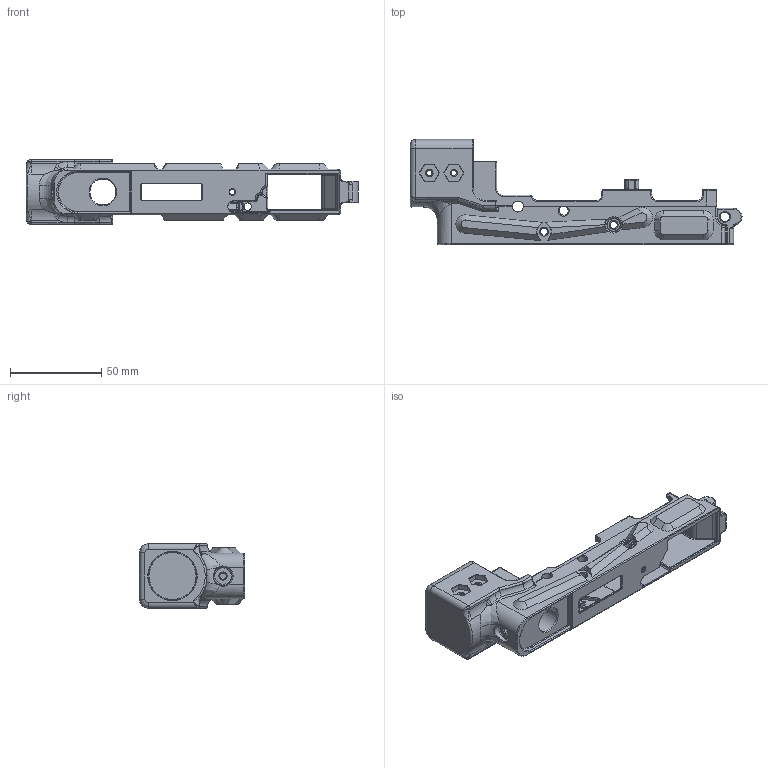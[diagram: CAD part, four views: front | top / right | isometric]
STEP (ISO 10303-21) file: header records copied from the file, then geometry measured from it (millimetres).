
FILE_DESCRIPTION(/* description */ (''),/* implementation_level */ '2;1');
FILE_NAME(/* name */ '38f86d36-2ef5-40c2-9561-66974e47ef92.stp',/* time_stamp */ '2019-03-05T10:23:56-05:00',/* author */ ('suzuki450ltr'),/* organization */ (''),/* preprocessor_version */ 'ST-DEVELOPER v17.2',/* originating_system */ 'Autodesk Translation Framework v7.6.0.251',/* authorisation */ '');
FILE_SCHEMA (('AUTOMOTIVE_DESIGN { 1 0 10303 214 3 1 1 }'));
Length unit declared in the file: millimetre
Products named in the file (3): vz61 skorpion v13; Default; Component2
Assembly tree (2 placements, depth 2):
  vz61 skorpion v13
    Default
    Component2
Bounding box: 181.54 x 57.49 x 35.48 mm (x, y, z)
Volume: 93568 mm3; surface area: 39927.2 mm2
Topology: 2 solids, 2 shells, 1064 faces, 2612 edges, 1510 vertices
Faces by surface type: cylinder 396, plane 242, bspline 206, torus 136, cone 56, sphere 28
Full cylindrical faces by diameter (mm): 1.5 x1, 2.946 x1, 3 x7, 3.5 x2, 3.556 x2, 3.95 x4, 4.039 x1, 4.978 x1, 5 x2, 6 x1, 8.75 x1, 10 x3, 14.173 x1, 25.75 x1, 26 x1
Entity records: 38440 total; most frequent: CARTESIAN_POINT 14109, ORIENTED_EDGE 5144, DIRECTION 5067, EDGE_CURVE 2572, AXIS2_PLACEMENT_3D 1998, VERTEX_POINT 1513, EDGE_LOOP 1119, LINE 1071
